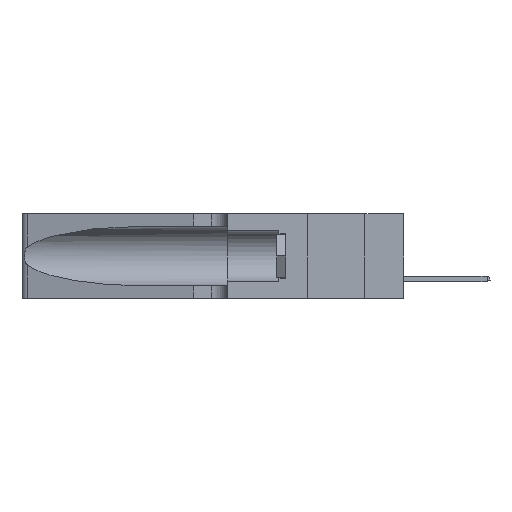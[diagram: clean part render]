
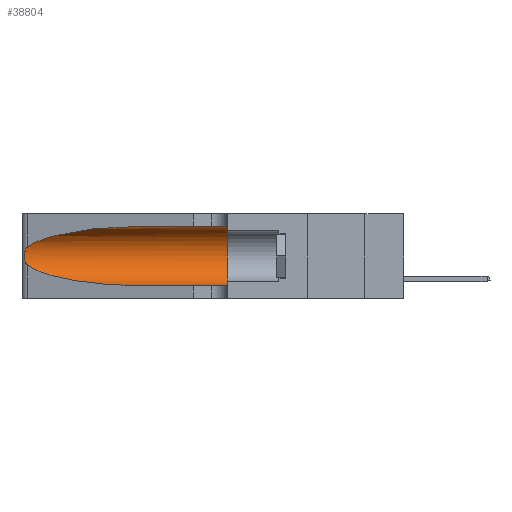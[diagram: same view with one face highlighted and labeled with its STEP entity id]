
A CAD part, left-side view. The second image highlights one B-rep face of the part: STEP entity #38804.
In plain terms, the highlighted cylindrical face has radius 3.308 mm (diameter 6.617 mm), a partial arc.
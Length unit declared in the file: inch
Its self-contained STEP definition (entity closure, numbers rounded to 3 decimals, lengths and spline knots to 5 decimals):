
#52 = LINE ( 'NONE', #8007, #27730 ) ;
#550 = VERTEX_POINT ( 'NONE', #29157 ) ;
#1051 = VECTOR ( 'NONE', #8855, 39.37008 ) ;
#1294 = CARTESIAN_POINT ( 'NONE',  ( 0.18966, 0.96281, 0.05475 ) ) ;
#1855 = CARTESIAN_POINT ( 'NONE',  ( 0.25487, 1.22718, 0.22369 ) ) ;
#3106 = EDGE_CURVE ( 'NONE', #550, #9775, #21629, .T. ) ;
#3648 = DIRECTION ( 'NONE',  ( 0., 0., -1. ) ) ;
#3839 = VERTEX_POINT ( 'NONE', #36033 ) ;
#5813 = CARTESIAN_POINT ( 'NONE',  ( 0.26017, 1.23833, 0.17102 ) ) ;
#6771 = FACE_OUTER_BOUND ( 'NONE', #8595, .T. ) ;
#6838 = CARTESIAN_POINT ( 'NONE',  ( 0.25487, 1.22718, 0.14631 ) ) ;
#7096 = VERTEX_POINT ( 'NONE', #32534 ) ;
#7284 = CARTESIAN_POINT ( 'NONE',  ( 0.25487, 1.22718, 0.22369 ) ) ;
#7502 = EDGE_CURVE ( 'NONE', #550, #35192, #9826, .T. ) ;
#7814 = CARTESIAN_POINT ( 'NONE',  ( 0.1305, 0.35, 0.185 ) ) ;
#8007 = CARTESIAN_POINT ( 'NONE',  ( 0.1305, 1.61858, 0.05475 ) ) ;
#8157 = ORIENTED_EDGE ( 'NONE', *, *, #3106, .T. ) ;
#8595 = EDGE_LOOP ( 'NONE', ( #8157, #10969, #36060, #26713, #23285, #38328 ) ) ;
#8855 = DIRECTION ( 'NONE',  ( 0., -1., 0. ) ) ;
#9775 = VERTEX_POINT ( 'NONE', #39112 ) ;
#9826 = LINE ( 'NONE', #35929, #1051 ) ;
#10182 = CARTESIAN_POINT ( 'NONE',  ( 0.25555, 1.22993, 0.14849 ) ) ;
#10683 = CARTESIAN_POINT ( 'NONE',  ( 0.2373, 1.15595, 0.08982 ) ) ;
#10969 = ORIENTED_EDGE ( 'NONE', *, *, #16096, .T. ) ;
#11040 = AXIS2_PLACEMENT_3D ( 'NONE', #38114, #28289, #3648 ) ;
#12587 = CYLINDRICAL_SURFACE ( 'NONE', #11040, 0.13025 ) ;
#13021 = CARTESIAN_POINT ( 'NONE',  ( 0.25639, 1.23186, 0.15144 ) ) ;
#13899 =( BOUNDED_CURVE ( )  B_SPLINE_CURVE ( 3, ( #29214, #10683, #1294, #16892 ),
 .UNSPECIFIED., .F., .T. ) 
 B_SPLINE_CURVE_WITH_KNOTS ( ( 4, 4 ),
 ( 3.44316, 4.71239 ),
 .UNSPECIFIED. ) 
 CURVE ( )  GEOMETRIC_REPRESENTATION_ITEM ( )  RATIONAL_B_SPLINE_CURVE ( ( 1., 0.87, 0.87, 1. ) ) 
 REPRESENTATION_ITEM ( '' )  );
#14005 = CARTESIAN_POINT ( 'NONE',  ( 0.25487, 1.22718, 0.14631 ) ) ;
#14010 = CARTESIAN_POINT ( 'NONE',  ( 0.26075, 1.23896, 0.19203 ) ) ;
#14049 = CARTESIAN_POINT ( 'NONE',  ( 0.2373, 1.15595, 0.28018 ) ) ;
#14114 = DIRECTION ( 'NONE',  ( 0., 1., 0. ) ) ;
#14405 = B_SPLINE_CURVE_WITH_KNOTS ( 'NONE', 3,
 ( #7284, #38467, #26584, #35892, #16975, #26312, #14010, #17946, #5813, #27442, #21466, #13021, #10182, #6838 ),
 .UNSPECIFIED., .F., .F.,
 ( 4, 2, 2, 2, 2, 2, 4 ),
 ( 0., 0.00027, 0.00053, 0.00107, 0.0016, 0.00187, 0.00214 ),
 .UNSPECIFIED. ) ;
#16096 = EDGE_CURVE ( 'NONE', #9775, #16837, #14405, .T. ) ;
#16837 = VERTEX_POINT ( 'NONE', #14005 ) ;
#16886 = CARTESIAN_POINT ( 'NONE',  ( 0.18966, 0.96281, 0.31525 ) ) ;
#16892 = CARTESIAN_POINT ( 'NONE',  ( 0.1305, 0.72297, 0.05475 ) ) ;
#16975 = CARTESIAN_POINT ( 'NONE',  ( 0.25854, 1.2359, 0.20912 ) ) ;
#17432 = CIRCLE ( 'NONE', #20864, 0.13025 ) ;
#17946 = CARTESIAN_POINT ( 'NONE',  ( 0.26075, 1.23896, 0.178 ) ) ;
#18450 = CARTESIAN_POINT ( 'NONE',  ( 0.1305, 0.35, 0.31525 ) ) ;
#20227 = DIRECTION ( 'NONE',  ( 0., 0., 1. ) ) ;
#20864 = AXIS2_PLACEMENT_3D ( 'NONE', #7814, #14114, #20227 ) ;
#21466 = CARTESIAN_POINT ( 'NONE',  ( 0.25789, 1.23486, 0.15765 ) ) ;
#21629 =( BOUNDED_CURVE ( )  B_SPLINE_CURVE ( 3, ( #39067, #16886, #14049, #1855 ),
 .UNSPECIFIED., .F., .F. ) 
 B_SPLINE_CURVE_WITH_KNOTS ( ( 4, 4 ),
 ( 1.5708, 2.84003 ),
 .UNSPECIFIED. ) 
 CURVE ( )  GEOMETRIC_REPRESENTATION_ITEM ( )  RATIONAL_B_SPLINE_CURVE ( ( 1., 0.87, 0.87, 1. ) ) 
 REPRESENTATION_ITEM ( '' )  );
#21852 = EDGE_CURVE ( 'NONE', #16837, #3839, #13899, .T. ) ;
#23285 = ORIENTED_EDGE ( 'NONE', *, *, #28841, .F. ) ;
#25989 = DIRECTION ( 'NONE',  ( 0., -1., 0. ) ) ;
#26312 = CARTESIAN_POINT ( 'NONE',  ( 0.26018, 1.23835, 0.19895 ) ) ;
#26584 = CARTESIAN_POINT ( 'NONE',  ( 0.25639, 1.23184, 0.21858 ) ) ;
#26713 = ORIENTED_EDGE ( 'NONE', *, *, #27494, .T. ) ;
#27442 = CARTESIAN_POINT ( 'NONE',  ( 0.25856, 1.23593, 0.16098 ) ) ;
#27494 = EDGE_CURVE ( 'NONE', #3839, #7096, #52, .T. ) ;
#27730 = VECTOR ( 'NONE', #25989, 39.37008 ) ;
#28289 = DIRECTION ( 'NONE',  ( 0., -1., 0. ) ) ;
#28841 = EDGE_CURVE ( 'NONE', #35192, #7096, #17432, .T. ) ;
#29157 = CARTESIAN_POINT ( 'NONE',  ( 0.1305, 0.72297, 0.31525 ) ) ;
#29214 = CARTESIAN_POINT ( 'NONE',  ( 0.25487, 1.22718, 0.14631 ) ) ;
#32534 = CARTESIAN_POINT ( 'NONE',  ( 0.1305, 0.35, 0.05475 ) ) ;
#35192 = VERTEX_POINT ( 'NONE', #18450 ) ;
#35892 = CARTESIAN_POINT ( 'NONE',  ( 0.25787, 1.23484, 0.2124 ) ) ;
#35929 = CARTESIAN_POINT ( 'NONE',  ( 0.1305, 1.61858, 0.31525 ) ) ;
#36033 = CARTESIAN_POINT ( 'NONE',  ( 0.1305, 0.72297, 0.05475 ) ) ;
#36060 = ORIENTED_EDGE ( 'NONE', *, *, #21852, .T. ) ;
#38114 = CARTESIAN_POINT ( 'NONE',  ( 0.1305, 1.61858, 0.185 ) ) ;
#38328 = ORIENTED_EDGE ( 'NONE', *, *, #7502, .F. ) ;
#38467 = CARTESIAN_POINT ( 'NONE',  ( 0.25555, 1.22994, 0.2215 ) ) ;
#38804 = ADVANCED_FACE ( 'NONE', ( #6771 ), #12587, .F. ) ;
#39067 = CARTESIAN_POINT ( 'NONE',  ( 0.1305, 0.72297, 0.31525 ) ) ;
#39112 = CARTESIAN_POINT ( 'NONE',  ( 0.25487, 1.22718, 0.22369 ) ) ;
